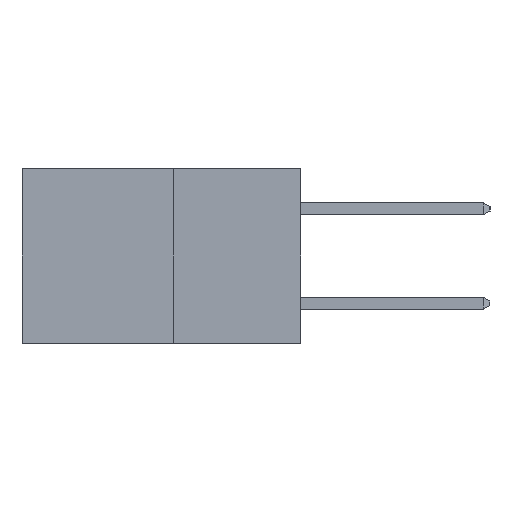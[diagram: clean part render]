
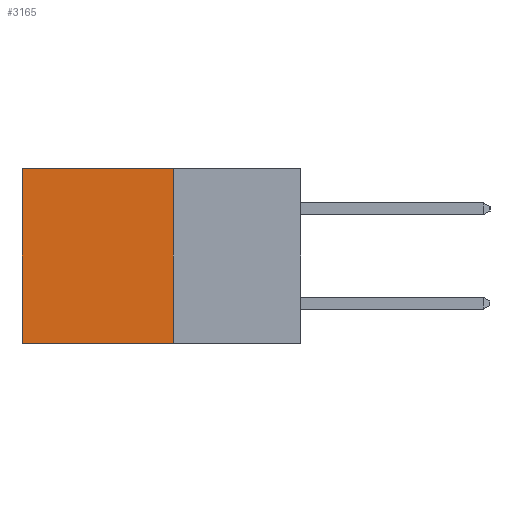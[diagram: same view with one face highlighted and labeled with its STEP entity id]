
A CAD part, left-side view. The second image highlights one B-rep face of the part: STEP entity #3165.
In plain terms, the highlighted planar face has unit normal (-1, 0, 0).
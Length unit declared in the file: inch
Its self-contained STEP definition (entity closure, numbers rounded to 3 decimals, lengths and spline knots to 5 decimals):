
#225 = AXIS2_PLACEMENT_3D ( 'NONE', #1492, #12577, #5844 ) ;
#323 = VECTOR ( 'NONE', #8103, 39.37008 ) ;
#1177 = PLANE ( 'NONE',  #225 ) ;
#1342 = LINE ( 'NONE', #12300, #6727 ) ;
#1492 = CARTESIAN_POINT ( 'NONE',  ( 0.277, 0.27, -0.37 ) ) ;
#1681 = CARTESIAN_POINT ( 'NONE',  ( 0.277, 0.59, 0. ) ) ;
#1729 = FACE_OUTER_BOUND ( 'NONE', #7492, .T. ) ;
#1792 = ORIENTED_EDGE ( 'NONE', *, *, #3327, .T. ) ;
#2105 = ORIENTED_EDGE ( 'NONE', *, *, #6127, .F. ) ;
#2794 = DIRECTION ( 'NONE',  ( 0., 1., 0. ) ) ;
#3165 = ADVANCED_FACE ( 'NONE', ( #1729 ), #1177, .F. ) ;
#3242 = VERTEX_POINT ( 'NONE', #4335 ) ;
#3327 = EDGE_CURVE ( 'NONE', #7965, #7718, #4886, .T. ) ;
#3808 = ORIENTED_EDGE ( 'NONE', *, *, #10661, .F. ) ;
#4335 = CARTESIAN_POINT ( 'NONE',  ( 0.277, 0.59, -0.37 ) ) ;
#4886 = LINE ( 'NONE', #7555, #12542 ) ;
#5078 = ORIENTED_EDGE ( 'NONE', *, *, #11338, .T. ) ;
#5844 = DIRECTION ( 'NONE',  ( 0., 0., -1. ) ) ;
#5882 = LINE ( 'NONE', #10775, #10607 ) ;
#6127 = EDGE_CURVE ( 'NONE', #7965, #11504, #1342, .T. ) ;
#6309 = CARTESIAN_POINT ( 'NONE',  ( 0.277, 0.27, -0.37 ) ) ;
#6727 = VECTOR ( 'NONE', #12410, 39.37008 ) ;
#7492 = EDGE_LOOP ( 'NONE', ( #5078, #3808, #2105, #1792 ) ) ;
#7555 = CARTESIAN_POINT ( 'NONE',  ( 0.277, 0.27, 0. ) ) ;
#7718 = VERTEX_POINT ( 'NONE', #1681 ) ;
#7965 = VERTEX_POINT ( 'NONE', #12700 ) ;
#8103 = DIRECTION ( 'NONE',  ( 0., 0., -1. ) ) ;
#8424 = LINE ( 'NONE', #11079, #323 ) ;
#8496 = DIRECTION ( 'NONE',  ( 0., 1., 0. ) ) ;
#10607 = VECTOR ( 'NONE', #2794, 39.37008 ) ;
#10661 = EDGE_CURVE ( 'NONE', #11504, #3242, #5882, .T. ) ;
#10775 = CARTESIAN_POINT ( 'NONE',  ( 0.277, 0.27, -0.37 ) ) ;
#11079 = CARTESIAN_POINT ( 'NONE',  ( 0.277, 0.59, -0.37 ) ) ;
#11338 = EDGE_CURVE ( 'NONE', #7718, #3242, #8424, .T. ) ;
#11504 = VERTEX_POINT ( 'NONE', #6309 ) ;
#12300 = CARTESIAN_POINT ( 'NONE',  ( 0.277, 0.27, -0.37 ) ) ;
#12410 = DIRECTION ( 'NONE',  ( 0., 0., -1. ) ) ;
#12542 = VECTOR ( 'NONE', #8496, 39.37008 ) ;
#12577 = DIRECTION ( 'NONE',  ( 1., 0., 0. ) ) ;
#12700 = CARTESIAN_POINT ( 'NONE',  ( 0.277, 0.27, 0. ) ) ;
